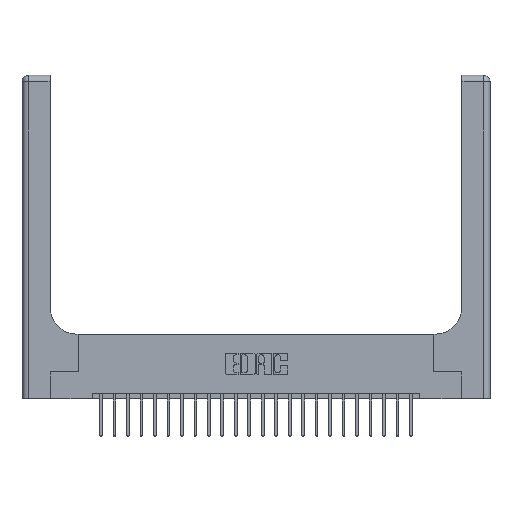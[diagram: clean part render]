
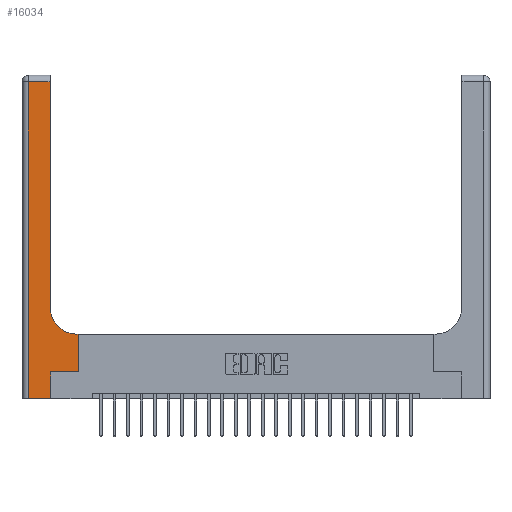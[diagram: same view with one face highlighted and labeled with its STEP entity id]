
A CAD part, top view. The second image highlights one B-rep face of the part: STEP entity #16034.
In plain terms, the highlighted planar face has unit normal (0, 0, 1).
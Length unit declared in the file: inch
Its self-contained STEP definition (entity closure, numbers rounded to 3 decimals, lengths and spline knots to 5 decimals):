
#65 = EDGE_CURVE ( 'NONE', #2236, #8862, #9964, .T. ) ;
#283 = VERTEX_POINT ( 'NONE', #5539 ) ;
#850 = CIRCLE ( 'NONE', #21077, 0.25 ) ;
#892 = DIRECTION ( 'NONE',  ( 1., 0., 0. ) ) ;
#1324 = VECTOR ( 'NONE', #22102, 39.37008 ) ;
#1366 = CARTESIAN_POINT ( 'NONE',  ( 0.528, 0.25, 0.37 ) ) ;
#1538 = VERTEX_POINT ( 'NONE', #7473 ) ;
#2005 = DIRECTION ( 'NONE',  ( 0., 1., 0. ) ) ;
#2236 = VERTEX_POINT ( 'NONE', #8457 ) ;
#2433 = DIRECTION ( 'NONE',  ( -1., 0., 0. ) ) ;
#2548 = VERTEX_POINT ( 'NONE', #15416 ) ;
#2982 = VECTOR ( 'NONE', #6566, 39.37008 ) ;
#2994 = CARTESIAN_POINT ( 'NONE',  ( 0.06, 3., 0.37 ) ) ;
#3576 = DIRECTION ( 'NONE',  ( -1., 0., 0. ) ) ;
#3613 = DIRECTION ( 'NONE',  ( 1., 0., 0. ) ) ;
#4465 = ORIENTED_EDGE ( 'NONE', *, *, #22307, .T. ) ;
#4515 = DIRECTION ( 'NONE',  ( 1., 0., 0. ) ) ;
#4543 = VERTEX_POINT ( 'NONE', #11747 ) ;
#4589 = EDGE_CURVE ( 'NONE', #1538, #20457, #18004, .T. ) ;
#5132 = EDGE_CURVE ( 'NONE', #283, #1538, #18266, .T. ) ;
#5539 = CARTESIAN_POINT ( 'NONE',  ( 0.06, 2.94, 0.37 ) ) ;
#5683 = ORIENTED_EDGE ( 'NONE', *, *, #4589, .T. ) ;
#6258 = AXIS2_PLACEMENT_3D ( 'NONE', #20414, #22079, #11274 ) ;
#6430 = ORIENTED_EDGE ( 'NONE', *, *, #14854, .T. ) ;
#6566 = DIRECTION ( 'NONE',  ( 0., -1., 0. ) ) ;
#6986 = LINE ( 'NONE', #10998, #1324 ) ;
#7225 = CARTESIAN_POINT ( 'NONE',  ( 0., 2.94, 0.37 ) ) ;
#7473 = CARTESIAN_POINT ( 'NONE',  ( 0.06, 0., 0.37 ) ) ;
#7783 = LINE ( 'NONE', #12852, #21025 ) ;
#8457 = CARTESIAN_POINT ( 'NONE',  ( 0.265, 0.25, 0.37 ) ) ;
#8579 = LINE ( 'NONE', #7225, #10529 ) ;
#8685 = LINE ( 'NONE', #13369, #17128 ) ;
#8862 = VERTEX_POINT ( 'NONE', #17878 ) ;
#8882 = VERTEX_POINT ( 'NONE', #14145 ) ;
#9964 = LINE ( 'NONE', #17050, #11920 ) ;
#10119 = DIRECTION ( 'NONE',  ( 0., 1., 0. ) ) ;
#10411 = EDGE_CURVE ( 'NONE', #8862, #8882, #14655, .T. ) ;
#10529 = VECTOR ( 'NONE', #3576, 39.37008 ) ;
#10623 = DIRECTION ( 'NONE',  ( 0., 0., -1. ) ) ;
#10805 = ORIENTED_EDGE ( 'NONE', *, *, #13710, .T. ) ;
#10998 = CARTESIAN_POINT ( 'NONE',  ( 0.26, 3., 0.37 ) ) ;
#11110 = VERTEX_POINT ( 'NONE', #18860 ) ;
#11274 = DIRECTION ( 'NONE',  ( -1., 0., 0. ) ) ;
#11298 = ORIENTED_EDGE ( 'NONE', *, *, #12148, .T. ) ;
#11747 = CARTESIAN_POINT ( 'NONE',  ( 0.26, 0.85, 0.37 ) ) ;
#11920 = VECTOR ( 'NONE', #892, 39.37008 ) ;
#11942 = ORIENTED_EDGE ( 'NONE', *, *, #10411, .T. ) ;
#12148 = EDGE_CURVE ( 'NONE', #4543, #11110, #6986, .T. ) ;
#12852 = CARTESIAN_POINT ( 'NONE',  ( 0.265, 0., 0.37 ) ) ;
#13369 = CARTESIAN_POINT ( 'NONE',  ( 0.26, 0.6, 0.37 ) ) ;
#13710 = EDGE_CURVE ( 'NONE', #8882, #2548, #8685, .T. ) ;
#14018 = CARTESIAN_POINT ( 'NONE',  ( 0.265, 0., 0.37 ) ) ;
#14145 = CARTESIAN_POINT ( 'NONE',  ( 0.528, 0.6, 0.37 ) ) ;
#14655 = LINE ( 'NONE', #1366, #21747 ) ;
#14854 = EDGE_CURVE ( 'NONE', #20457, #2236, #7783, .T. ) ;
#15330 = FACE_OUTER_BOUND ( 'NONE', #22956, .T. ) ;
#15416 = CARTESIAN_POINT ( 'NONE',  ( 0.51, 0.6, 0.37 ) ) ;
#15419 = CARTESIAN_POINT ( 'NONE',  ( 0., 0., 0.37 ) ) ;
#16034 = ADVANCED_FACE ( 'NONE', ( #15330 ), #18632, .F. ) ;
#17050 = CARTESIAN_POINT ( 'NONE',  ( 0.265, 0.25, 0.37 ) ) ;
#17128 = VECTOR ( 'NONE', #2433, 39.37008 ) ;
#17878 = CARTESIAN_POINT ( 'NONE',  ( 0.528, 0.25, 0.37 ) ) ;
#17965 = EDGE_CURVE ( 'NONE', #2548, #4543, #850, .T. ) ;
#18004 = LINE ( 'NONE', #15419, #21667 ) ;
#18266 = LINE ( 'NONE', #2994, #2982 ) ;
#18632 = PLANE ( 'NONE',  #6258 ) ;
#18860 = CARTESIAN_POINT ( 'NONE',  ( 0.26, 2.94, 0.37 ) ) ;
#18958 = ORIENTED_EDGE ( 'NONE', *, *, #65, .T. ) ;
#19564 = CARTESIAN_POINT ( 'NONE',  ( 0.51, 0.85, 0.37 ) ) ;
#19882 = ORIENTED_EDGE ( 'NONE', *, *, #17965, .T. ) ;
#20414 = CARTESIAN_POINT ( 'NONE',  ( 0., 3., 0.37 ) ) ;
#20457 = VERTEX_POINT ( 'NONE', #14018 ) ;
#21025 = VECTOR ( 'NONE', #2005, 39.37008 ) ;
#21077 = AXIS2_PLACEMENT_3D ( 'NONE', #19564, #10623, #3613 ) ;
#21667 = VECTOR ( 'NONE', #4515, 39.37008 ) ;
#21747 = VECTOR ( 'NONE', #10119, 39.37008 ) ;
#22079 = DIRECTION ( 'NONE',  ( 0., 0., -1. ) ) ;
#22102 = DIRECTION ( 'NONE',  ( 0., 1., 0. ) ) ;
#22307 = EDGE_CURVE ( 'NONE', #11110, #283, #8579, .T. ) ;
#22698 = ORIENTED_EDGE ( 'NONE', *, *, #5132, .T. ) ;
#22956 = EDGE_LOOP ( 'NONE', ( #11298, #4465, #22698, #5683, #6430, #18958, #11942, #10805, #19882 ) ) ;
